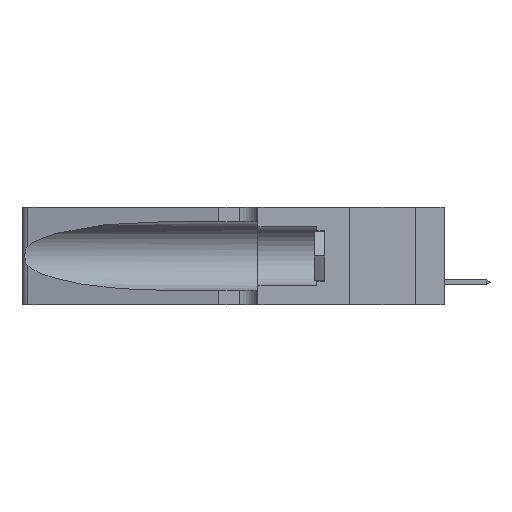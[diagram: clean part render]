
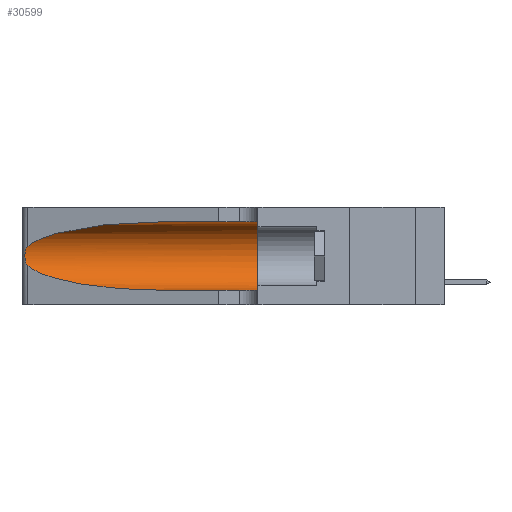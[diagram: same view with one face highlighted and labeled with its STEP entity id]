
A CAD part, left-side view. The second image highlights one B-rep face of the part: STEP entity #30599.
In plain terms, the highlighted cylindrical face has radius 3.308 mm (diameter 6.617 mm), a partial arc.
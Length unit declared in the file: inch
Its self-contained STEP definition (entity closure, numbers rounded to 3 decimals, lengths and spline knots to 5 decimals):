
#18 = B_SPLINE_CURVE_WITH_KNOTS ( 'NONE', 3,
 ( #9222, #16046, #25649, #39362, #12642, #5183, #32662, #22391, #32358, #15603, #12347, #42762, #36151, #22549 ),
 .UNSPECIFIED., .F., .F.,
 ( 4, 2, 2, 2, 2, 2, 4 ),
 ( 0., 0.00027, 0.00053, 0.00107, 0.0016, 0.00187, 0.00214 ),
 .UNSPECIFIED. ) ;
#1120 = CARTESIAN_POINT ( 'NONE',  ( 0.1305, 0.35, 0.185 ) ) ;
#5183 = CARTESIAN_POINT ( 'NONE',  ( 0.26018, 1.23835, 0.19895 ) ) ;
#5626 = CARTESIAN_POINT ( 'NONE',  ( 0.25487, 1.22718, 0.14631 ) ) ;
#5796 = AXIS2_PLACEMENT_3D ( 'NONE', #18523, #21611, #12024 ) ;
#6037 = CARTESIAN_POINT ( 'NONE',  ( 0.18966, 0.96281, 0.31525 ) ) ;
#7370 = CYLINDRICAL_SURFACE ( 'NONE', #5796, 0.13025 ) ;
#7977 = VECTOR ( 'NONE', #36925, 39.37008 ) ;
#8468 = FACE_OUTER_BOUND ( 'NONE', #42961, .T. ) ;
#9222 = CARTESIAN_POINT ( 'NONE',  ( 0.25487, 1.22718, 0.22369 ) ) ;
#9225 = VECTOR ( 'NONE', #41008, 39.37008 ) ;
#10693 = CARTESIAN_POINT ( 'NONE',  ( 0.1305, 0.35, 0.05475 ) ) ;
#10720 = CARTESIAN_POINT ( 'NONE',  ( 0.25487, 1.22718, 0.22369 ) ) ;
#12024 = DIRECTION ( 'NONE',  ( 0., 0., -1. ) ) ;
#12347 = CARTESIAN_POINT ( 'NONE',  ( 0.25789, 1.23486, 0.15765 ) ) ;
#12642 = CARTESIAN_POINT ( 'NONE',  ( 0.25854, 1.2359, 0.20912 ) ) ;
#13180 = EDGE_CURVE ( 'NONE', #28212, #42332, #29734, .T. ) ;
#13226 = EDGE_CURVE ( 'NONE', #42931, #38190, #39794, .T. ) ;
#15016 = DIRECTION ( 'NONE',  ( 0., 0., 1. ) ) ;
#15279 = CARTESIAN_POINT ( 'NONE',  ( 0.1305, 0.35, 0.31525 ) ) ;
#15458 = EDGE_CURVE ( 'NONE', #26153, #28212, #18, .T. ) ;
#15603 = CARTESIAN_POINT ( 'NONE',  ( 0.25856, 1.23593, 0.16098 ) ) ;
#15668 = VERTEX_POINT ( 'NONE', #10693 ) ;
#16046 = CARTESIAN_POINT ( 'NONE',  ( 0.25555, 1.22994, 0.2215 ) ) ;
#16593 = CARTESIAN_POINT ( 'NONE',  ( 0.25487, 1.22718, 0.22369 ) ) ;
#18523 = CARTESIAN_POINT ( 'NONE',  ( 0.1305, 1.61858, 0.185 ) ) ;
#19237 = EDGE_CURVE ( 'NONE', #38190, #15668, #35569, .T. ) ;
#20011 = CARTESIAN_POINT ( 'NONE',  ( 0.25487, 1.22718, 0.14631 ) ) ;
#21269 = CARTESIAN_POINT ( 'NONE',  ( 0.1305, 0.72297, 0.05475 ) ) ;
#21611 = DIRECTION ( 'NONE',  ( 0., -1., 0. ) ) ;
#22391 = CARTESIAN_POINT ( 'NONE',  ( 0.26075, 1.23896, 0.178 ) ) ;
#22549 = CARTESIAN_POINT ( 'NONE',  ( 0.25487, 1.22718, 0.14631 ) ) ;
#23193 = ORIENTED_EDGE ( 'NONE', *, *, #13180, .T. ) ;
#23263 = EDGE_CURVE ( 'NONE', #42931, #26153, #42120, .T. ) ;
#23497 = CARTESIAN_POINT ( 'NONE',  ( 0.1305, 1.61858, 0.31525 ) ) ;
#24221 = AXIS2_PLACEMENT_3D ( 'NONE', #1120, #24918, #15016 ) ;
#24314 = ORIENTED_EDGE ( 'NONE', *, *, #19237, .F. ) ;
#24913 = ORIENTED_EDGE ( 'NONE', *, *, #42810, .T. ) ;
#24918 = DIRECTION ( 'NONE',  ( 0., 1., 0. ) ) ;
#25649 = CARTESIAN_POINT ( 'NONE',  ( 0.25639, 1.23184, 0.21858 ) ) ;
#26153 = VERTEX_POINT ( 'NONE', #10720 ) ;
#26727 = CARTESIAN_POINT ( 'NONE',  ( 0.18966, 0.96281, 0.05475 ) ) ;
#28212 = VERTEX_POINT ( 'NONE', #20011 ) ;
#28416 = ORIENTED_EDGE ( 'NONE', *, *, #13226, .F. ) ;
#29734 =( BOUNDED_CURVE ( )  B_SPLINE_CURVE ( 3, ( #5626, #30959, #26727, #40600 ),
 .UNSPECIFIED., .F., .F. ) 
 B_SPLINE_CURVE_WITH_KNOTS ( ( 4, 4 ),
 ( 3.44316, 4.71239 ),
 .UNSPECIFIED. ) 
 CURVE ( )  GEOMETRIC_REPRESENTATION_ITEM ( )  RATIONAL_B_SPLINE_CURVE ( ( 1., 0.87, 0.87, 1. ) ) 
 REPRESENTATION_ITEM ( '' )  );
#30599 = ADVANCED_FACE ( 'NONE', ( #8468 ), #7370, .F. ) ;
#30656 = CARTESIAN_POINT ( 'NONE',  ( 0.2373, 1.15595, 0.28018 ) ) ;
#30959 = CARTESIAN_POINT ( 'NONE',  ( 0.2373, 1.15595, 0.08982 ) ) ;
#32358 = CARTESIAN_POINT ( 'NONE',  ( 0.26017, 1.23833, 0.17102 ) ) ;
#32662 = CARTESIAN_POINT ( 'NONE',  ( 0.26075, 1.23896, 0.19203 ) ) ;
#34106 = LINE ( 'NONE', #40860, #9225 ) ;
#34283 = CARTESIAN_POINT ( 'NONE',  ( 0.1305, 0.72297, 0.31525 ) ) ;
#35569 = CIRCLE ( 'NONE', #24221, 0.13025 ) ;
#36151 = CARTESIAN_POINT ( 'NONE',  ( 0.25555, 1.22993, 0.14849 ) ) ;
#36756 = ORIENTED_EDGE ( 'NONE', *, *, #15458, .T. ) ;
#36925 = DIRECTION ( 'NONE',  ( 0., -1., 0. ) ) ;
#38190 = VERTEX_POINT ( 'NONE', #15279 ) ;
#38991 = ORIENTED_EDGE ( 'NONE', *, *, #23263, .T. ) ;
#39362 = CARTESIAN_POINT ( 'NONE',  ( 0.25787, 1.23484, 0.2124 ) ) ;
#39794 = LINE ( 'NONE', #23497, #7977 ) ;
#40600 = CARTESIAN_POINT ( 'NONE',  ( 0.1305, 0.72297, 0.05475 ) ) ;
#40860 = CARTESIAN_POINT ( 'NONE',  ( 0.1305, 1.61858, 0.05475 ) ) ;
#41008 = DIRECTION ( 'NONE',  ( 0., -1., 0. ) ) ;
#42120 =( BOUNDED_CURVE ( )  B_SPLINE_CURVE ( 3, ( #43168, #6037, #30656, #16593 ),
 .UNSPECIFIED., .F., .T. ) 
 B_SPLINE_CURVE_WITH_KNOTS ( ( 4, 4 ),
 ( 1.5708, 2.84003 ),
 .UNSPECIFIED. ) 
 CURVE ( )  GEOMETRIC_REPRESENTATION_ITEM ( )  RATIONAL_B_SPLINE_CURVE ( ( 1., 0.87, 0.87, 1. ) ) 
 REPRESENTATION_ITEM ( '' )  );
#42332 = VERTEX_POINT ( 'NONE', #21269 ) ;
#42762 = CARTESIAN_POINT ( 'NONE',  ( 0.25639, 1.23186, 0.15144 ) ) ;
#42810 = EDGE_CURVE ( 'NONE', #42332, #15668, #34106, .T. ) ;
#42931 = VERTEX_POINT ( 'NONE', #34283 ) ;
#42961 = EDGE_LOOP ( 'NONE', ( #38991, #36756, #23193, #24913, #24314, #28416 ) ) ;
#43168 = CARTESIAN_POINT ( 'NONE',  ( 0.1305, 0.72297, 0.31525 ) ) ;
